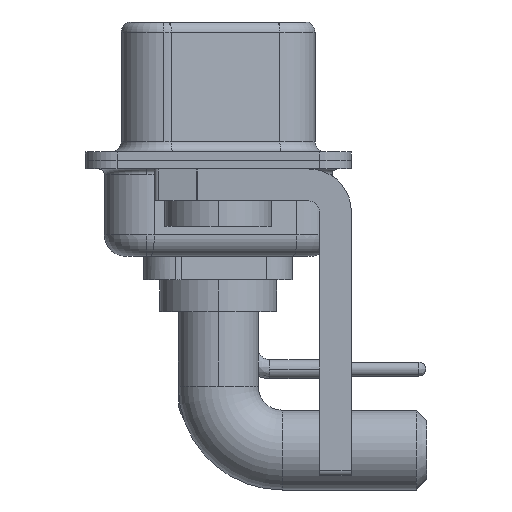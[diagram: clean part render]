
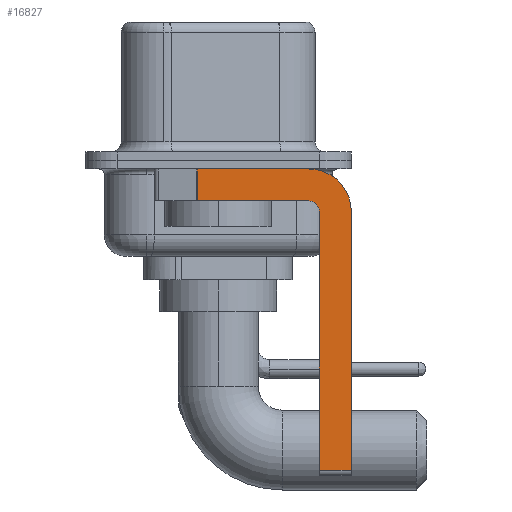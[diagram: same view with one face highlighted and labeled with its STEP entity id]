
A CAD part, left-side view. The second image highlights one B-rep face of the part: STEP entity #16827.
In plain terms, the highlighted planar face has unit normal (-1, 0, 0).
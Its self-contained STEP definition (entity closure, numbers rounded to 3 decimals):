
#85 = DIRECTION ( 'NONE',  ( 0., 0., -1. ) ) ;
#486 = EDGE_CURVE ( 'NONE', #16943, #2711, #26121, .T. ) ;
#634 = LINE ( 'NONE', #3156, #17603 ) ;
#783 = DIRECTION ( 'NONE',  ( 0., 0., -1. ) ) ;
#1077 = DIRECTION ( 'NONE',  ( -1., 0., 0. ) ) ;
#1904 = CARTESIAN_POINT ( 'NONE',  ( -2.9, -4.75, -2.4 ) ) ;
#2442 = ORIENTED_EDGE ( 'NONE', *, *, #25470, .T. ) ;
#2711 = VERTEX_POINT ( 'NONE', #6932 ) ;
#2902 = VERTEX_POINT ( 'NONE', #23030 ) ;
#2994 = DIRECTION ( 'NONE',  ( 1., 0., 0. ) ) ;
#3156 = CARTESIAN_POINT ( 'NONE',  ( -2.9, 0.978, -1.9 ) ) ;
#4059 = EDGE_CURVE ( 'NONE', #2902, #2711, #634, .T. ) ;
#4852 = ORIENTED_EDGE ( 'NONE', *, *, #14408, .F. ) ;
#5094 = VECTOR ( 'NONE', #17973, 1000. ) ;
#5357 = VECTOR ( 'NONE', #21607, 1000. ) ;
#5909 = EDGE_CURVE ( 'NONE', #17123, #12837, #26293, .T. ) ;
#6024 = AXIS2_PLACEMENT_3D ( 'NONE', #23228, #6549, #19559 ) ;
#6549 = DIRECTION ( 'NONE',  ( 1., 0., 0. ) ) ;
#6682 = ORIENTED_EDGE ( 'NONE', *, *, #5909, .F. ) ;
#6932 = CARTESIAN_POINT ( 'NONE',  ( -2.9, 0.978, -1.9 ) ) ;
#7513 = VERTEX_POINT ( 'NONE', #10339 ) ;
#8391 = VECTOR ( 'NONE', #11213, 1000. ) ;
#8626 = VECTOR ( 'NONE', #11839, 1000. ) ;
#9277 = VECTOR ( 'NONE', #85, 1000. ) ;
#9632 = DIRECTION ( 'NONE',  ( 0., 0., 1. ) ) ;
#10021 = LINE ( 'NONE', #14354, #8626 ) ;
#10033 = ORIENTED_EDGE ( 'NONE', *, *, #17448, .F. ) ;
#10339 = CARTESIAN_POINT ( 'NONE',  ( -2.9, -6.25, -2.4 ) ) ;
#11091 = ORIENTED_EDGE ( 'NONE', *, *, #486, .F. ) ;
#11213 = DIRECTION ( 'NONE',  ( 0., -1., 0. ) ) ;
#11839 = DIRECTION ( 'NONE',  ( 0., -1., 0. ) ) ;
#11900 = CARTESIAN_POINT ( 'NONE',  ( -2.9, -4.25, -0.4 ) ) ;
#12837 = VERTEX_POINT ( 'NONE', #1904 ) ;
#12900 = ORIENTED_EDGE ( 'NONE', *, *, #19763, .F. ) ;
#13053 = CARTESIAN_POINT ( 'NONE',  ( -2.9, -4.25, -14.55 ) ) ;
#13081 = CARTESIAN_POINT ( 'NONE',  ( -2.9, -4.25, -1.9 ) ) ;
#14354 = CARTESIAN_POINT ( 'NONE',  ( -2.9, 3., -0.4 ) ) ;
#14408 = EDGE_CURVE ( 'NONE', #22160, #7513, #18104, .T. ) ;
#14879 = VERTEX_POINT ( 'NONE', #23187 ) ;
#15622 = CIRCLE ( 'NONE', #19213, 0.5 ) ;
#16827 = ADVANCED_FACE ( 'NONE', ( #20501 ), #18384, .F. ) ;
#16943 = VERTEX_POINT ( 'NONE', #24524 ) ;
#17123 = VERTEX_POINT ( 'NONE', #17185 ) ;
#17185 = CARTESIAN_POINT ( 'NONE',  ( -2.9, -4.75, -14.55 ) ) ;
#17448 = EDGE_CURVE ( 'NONE', #12837, #16943, #15622, .T. ) ;
#17574 = CARTESIAN_POINT ( 'NONE',  ( -2.9, -6.25, -2.4 ) ) ;
#17603 = VECTOR ( 'NONE', #783, 1000. ) ;
#17699 = CARTESIAN_POINT ( 'NONE',  ( -2.9, -4.75, -14.8 ) ) ;
#17973 = DIRECTION ( 'NONE',  ( 0., 0., 1. ) ) ;
#18104 = CIRCLE ( 'NONE', #6024, 2. ) ;
#18384 = PLANE ( 'NONE',  #18743 ) ;
#18743 = AXIS2_PLACEMENT_3D ( 'NONE', #26550, #2994, #26973 ) ;
#19143 = LINE ( 'NONE', #17574, #9277 ) ;
#19213 = AXIS2_PLACEMENT_3D ( 'NONE', #22370, #1077, #9632 ) ;
#19559 = DIRECTION ( 'NONE',  ( 0., 0., -1. ) ) ;
#19763 = EDGE_CURVE ( 'NONE', #2902, #22160, #10021, .T. ) ;
#20501 = FACE_OUTER_BOUND ( 'NONE', #23303, .T. ) ;
#21448 = LINE ( 'NONE', #13053, #8391 ) ;
#21607 = DIRECTION ( 'NONE',  ( 0., 1., 0. ) ) ;
#22160 = VERTEX_POINT ( 'NONE', #11900 ) ;
#22370 = CARTESIAN_POINT ( 'NONE',  ( -2.9, -4.25, -2.4 ) ) ;
#23030 = CARTESIAN_POINT ( 'NONE',  ( -2.9, 0.978, -0.4 ) ) ;
#23187 = CARTESIAN_POINT ( 'NONE',  ( -2.9, -6.25, -14.55 ) ) ;
#23228 = CARTESIAN_POINT ( 'NONE',  ( -2.9, -4.25, -2.4 ) ) ;
#23303 = EDGE_LOOP ( 'NONE', ( #12900, #23838, #11091, #10033, #6682, #2442, #26876, #4852 ) ) ;
#23838 = ORIENTED_EDGE ( 'NONE', *, *, #4059, .T. ) ;
#24524 = CARTESIAN_POINT ( 'NONE',  ( -2.9, -4.25, -1.9 ) ) ;
#25470 = EDGE_CURVE ( 'NONE', #17123, #14879, #21448, .T. ) ;
#25747 = EDGE_CURVE ( 'NONE', #7513, #14879, #19143, .T. ) ;
#26121 = LINE ( 'NONE', #13081, #5357 ) ;
#26293 = LINE ( 'NONE', #17699, #5094 ) ;
#26550 = CARTESIAN_POINT ( 'NONE',  ( -2.9, -4.25, -2.4 ) ) ;
#26876 = ORIENTED_EDGE ( 'NONE', *, *, #25747, .F. ) ;
#26973 = DIRECTION ( 'NONE',  ( 0., 0., -1. ) ) ;
